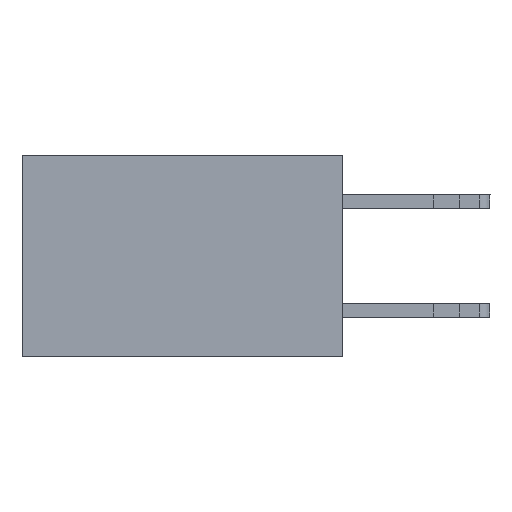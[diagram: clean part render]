
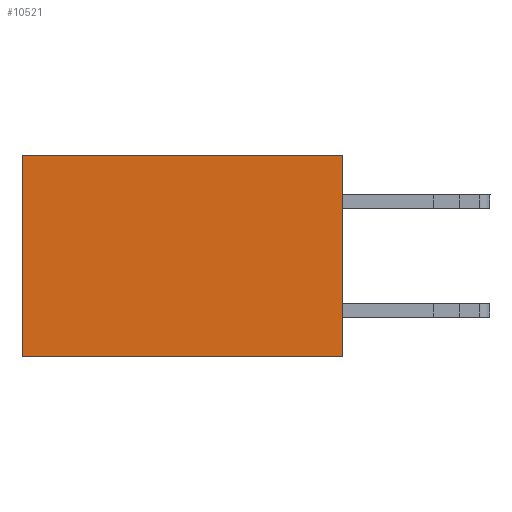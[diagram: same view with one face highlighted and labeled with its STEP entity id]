
A CAD part, left-side view. The second image highlights one B-rep face of the part: STEP entity #10521.
In plain terms, the highlighted planar face has unit normal (-1, 0, 0).
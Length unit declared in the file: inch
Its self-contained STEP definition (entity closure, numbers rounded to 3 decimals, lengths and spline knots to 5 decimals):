
#926 = DIRECTION ( 'NONE',  ( 0., 1., 0. ) ) ;
#1311 = PLANE ( 'NONE',  #11733 ) ;
#1446 = EDGE_CURVE ( 'NONE', #13175, #10699, #12671, .T. ) ;
#2266 = CARTESIAN_POINT ( 'NONE',  ( 0.277, 0.59, 0. ) ) ;
#2536 = DIRECTION ( 'NONE',  ( 0., 1., 0. ) ) ;
#3233 = ORIENTED_EDGE ( 'NONE', *, *, #5422, .F. ) ;
#4239 = VECTOR ( 'NONE', #2536, 39.37008 ) ;
#4947 = DIRECTION ( 'NONE',  ( 0., 0., -1. ) ) ;
#5422 = EDGE_CURVE ( 'NONE', #12380, #10699, #8824, .T. ) ;
#6018 = CARTESIAN_POINT ( 'NONE',  ( 0.277, 0., -0.37 ) ) ;
#6113 = ORIENTED_EDGE ( 'NONE', *, *, #7995, .T. ) ;
#6385 = CARTESIAN_POINT ( 'NONE',  ( 0.277, 0.59, -0.37 ) ) ;
#6885 = CARTESIAN_POINT ( 'NONE',  ( 0.277, 0.59, -0.37 ) ) ;
#7337 = EDGE_LOOP ( 'NONE', ( #10513, #3233, #11933, #6113 ) ) ;
#7522 = DIRECTION ( 'NONE',  ( 0., 0., -1. ) ) ;
#7912 = CARTESIAN_POINT ( 'NONE',  ( 0.277, 0., -0.37 ) ) ;
#7995 = EDGE_CURVE ( 'NONE', #13994, #13175, #8995, .T. ) ;
#8307 = CARTESIAN_POINT ( 'NONE',  ( 0.277, 0., 0. ) ) ;
#8824 = LINE ( 'NONE', #6018, #10698 ) ;
#8995 = LINE ( 'NONE', #14175, #4239 ) ;
#10513 = ORIENTED_EDGE ( 'NONE', *, *, #1446, .T. ) ;
#10521 = ADVANCED_FACE ( 'NONE', ( #10621 ), #1311, .F. ) ;
#10621 = FACE_OUTER_BOUND ( 'NONE', #7337, .T. ) ;
#10698 = VECTOR ( 'NONE', #926, 39.37008 ) ;
#10699 = VERTEX_POINT ( 'NONE', #6885 ) ;
#11500 = VECTOR ( 'NONE', #4947, 39.37008 ) ;
#11522 = CARTESIAN_POINT ( 'NONE',  ( 0.277, 0., -0.37 ) ) ;
#11684 = LINE ( 'NONE', #11522, #13448 ) ;
#11733 = AXIS2_PLACEMENT_3D ( 'NONE', #7912, #11982, #15819 ) ;
#11933 = ORIENTED_EDGE ( 'NONE', *, *, #16108, .F. ) ;
#11982 = DIRECTION ( 'NONE',  ( 1., 0., 0. ) ) ;
#12380 = VERTEX_POINT ( 'NONE', #13009 ) ;
#12671 = LINE ( 'NONE', #6385, #11500 ) ;
#13009 = CARTESIAN_POINT ( 'NONE',  ( 0.277, 0., -0.37 ) ) ;
#13175 = VERTEX_POINT ( 'NONE', #2266 ) ;
#13448 = VECTOR ( 'NONE', #7522, 39.37008 ) ;
#13994 = VERTEX_POINT ( 'NONE', #8307 ) ;
#14175 = CARTESIAN_POINT ( 'NONE',  ( 0.277, 0., 0. ) ) ;
#15819 = DIRECTION ( 'NONE',  ( 0., 0., -1. ) ) ;
#16108 = EDGE_CURVE ( 'NONE', #13994, #12380, #11684, .T. ) ;
